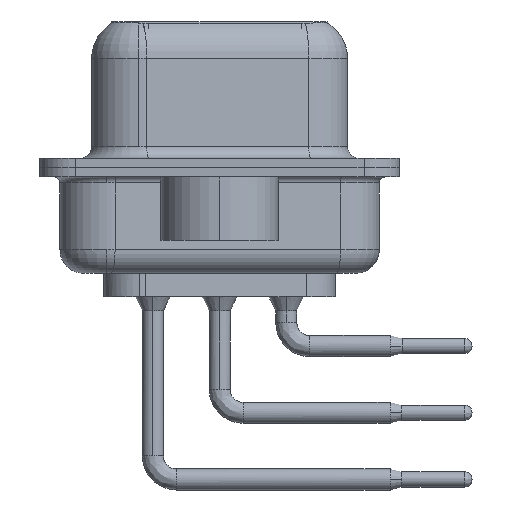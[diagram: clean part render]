
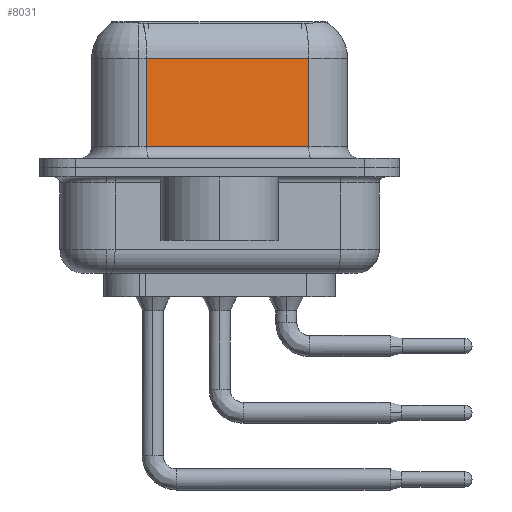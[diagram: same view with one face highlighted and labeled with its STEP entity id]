
A CAD part, left-side view. The second image highlights one B-rep face of the part: STEP entity #8031.
In plain terms, the highlighted planar face has unit normal (-0.985, -0.174, 0).
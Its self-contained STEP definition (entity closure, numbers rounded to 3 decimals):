
#2233 = ORIENTED_EDGE ( 'NONE', *, *, #2291, .T. ) ;
#2280 = CARTESIAN_POINT ( 'NONE',  ( 5.647, -3.797, 6.4 ) ) ;
#2291 = EDGE_CURVE ( 'NONE', #29208, #13194, #12745, .T. ) ;
#3059 = ORIENTED_EDGE ( 'NONE', *, *, #17907, .T. ) ;
#3251 = FACE_OUTER_BOUND ( 'NONE', #23131, .T. ) ;
#6896 = LINE ( 'NONE', #27295, #12953 ) ;
#8031 = ADVANCED_FACE ( 'NONE', ( #3251 ), #33114, .F. ) ;
#8688 = ORIENTED_EDGE ( 'NONE', *, *, #16603, .F. ) ;
#9537 = CARTESIAN_POINT ( 'NONE',  ( 5.647, -3.797, 0.9 ) ) ;
#9973 = DIRECTION ( 'NONE',  ( -0.174, 0.985, 0. ) ) ;
#10395 = VERTEX_POINT ( 'NONE', #9537 ) ;
#11935 = DIRECTION ( 'NONE',  ( 0., 0., -1. ) ) ;
#12745 = LINE ( 'NONE', #27046, #26389 ) ;
#12953 = VECTOR ( 'NONE', #14470, 1000. ) ;
#13194 = VERTEX_POINT ( 'NONE', #16035 ) ;
#13257 = CARTESIAN_POINT ( 'NONE',  ( 4.43, 3.103, 4.65 ) ) ;
#14113 = ORIENTED_EDGE ( 'NONE', *, *, #20324, .T. ) ;
#14470 = DIRECTION ( 'NONE',  ( 0.174, -0.985, 0. ) ) ;
#16035 = CARTESIAN_POINT ( 'NONE',  ( 4.43, 3.103, 0.9 ) ) ;
#16603 = EDGE_CURVE ( 'NONE', #33161, #10395, #26269, .T. ) ;
#17907 = EDGE_CURVE ( 'NONE', #13194, #10395, #6896, .T. ) ;
#18431 = DIRECTION ( 'NONE',  ( -0.174, 0.985, 0. ) ) ;
#20324 = EDGE_CURVE ( 'NONE', #33161, #29208, #25633, .T. ) ;
#20743 = CARTESIAN_POINT ( 'NONE',  ( 5.647, -3.797, 4.65 ) ) ;
#22156 = CARTESIAN_POINT ( 'NONE',  ( 5.647, -3.797, 6.4 ) ) ;
#23131 = EDGE_LOOP ( 'NONE', ( #8688, #14113, #2233, #3059 ) ) ;
#25376 = DIRECTION ( 'NONE',  ( 0.985, 0.174, 0. ) ) ;
#25633 = LINE ( 'NONE', #31230, #31722 ) ;
#26269 = LINE ( 'NONE', #22156, #31547 ) ;
#26389 = VECTOR ( 'NONE', #32557, 1000. ) ;
#27046 = CARTESIAN_POINT ( 'NONE',  ( 4.43, 3.103, 6.4 ) ) ;
#27295 = CARTESIAN_POINT ( 'NONE',  ( 5.647, -3.797, 0.9 ) ) ;
#29095 = AXIS2_PLACEMENT_3D ( 'NONE', #2280, #25376, #9973 ) ;
#29208 = VERTEX_POINT ( 'NONE', #13257 ) ;
#31230 = CARTESIAN_POINT ( 'NONE',  ( 5.647, -3.797, 4.65 ) ) ;
#31547 = VECTOR ( 'NONE', #11935, 1000. ) ;
#31722 = VECTOR ( 'NONE', #18431, 1000. ) ;
#32557 = DIRECTION ( 'NONE',  ( 0., 0., -1. ) ) ;
#33114 = PLANE ( 'NONE',  #29095 ) ;
#33161 = VERTEX_POINT ( 'NONE', #20743 ) ;
